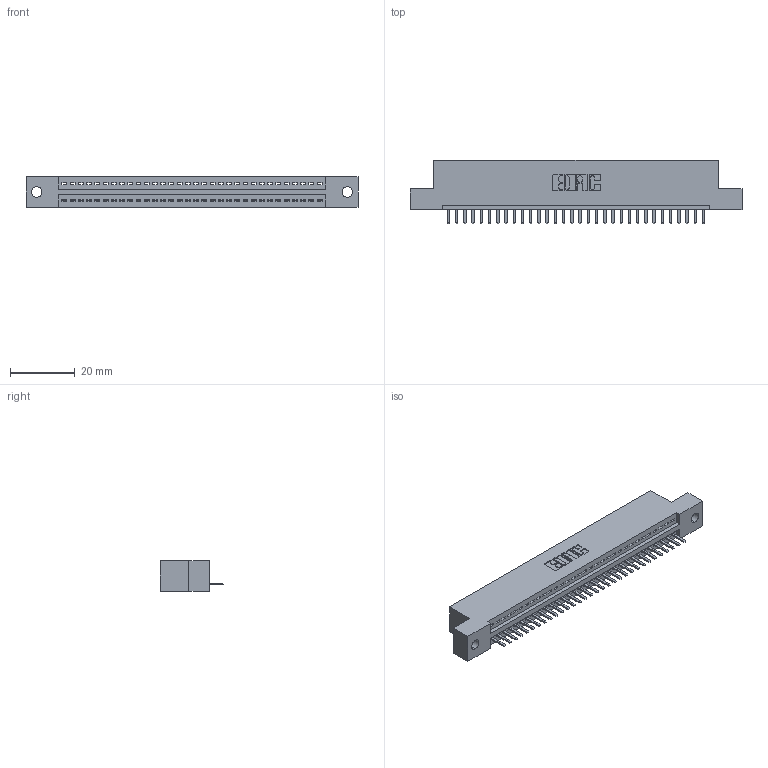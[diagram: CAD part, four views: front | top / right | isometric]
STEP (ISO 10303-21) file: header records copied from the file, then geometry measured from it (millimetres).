
FILE_DESCRIPTION (( 'STEP AP203' ), '1' );
FILE_NAME ('345-032-520-102.STEP', '2018-08-24T04:38:52', ( '' ), ( '' ), 'SwSTEP 2.0', 'SolidWorks 2016', '' );
FILE_SCHEMA (( 'CONFIG_CONTROL_DESIGN' ));
Length unit declared in the file: inch
Products named in the file (3): 345 Part_Flush Mounting Lugs - 0.128 Dia; 345-292-001_345-293-120; 345-032-520-102
Assembly tree (33 placements, depth 2):
  345-032-520-102
    345 Part_Flush Mounting Lugs - 0.128 Dia
    345-292-001_345-293-120  x32
Bounding box: 102.49 x 19.68 x 9.4 mm (x, y, z)
Volume: 9523.9 mm3; surface area: 11947.8 mm2
Topology: 33 solids, 33 shells, 2110 faces, 6229 edges, 4066 vertices
Faces by surface type: plane 1424, cylinder 686
Entity records: 25547 total; most frequent: CARTESIAN_POINT 4444, ORIENTED_EDGE 4398, DIRECTION 3883, EDGE_CURVE 2199, VECTOR 1935, LINE 1935, VERTEX_POINT 1462, AXIS2_PLACEMENT_3D 974
